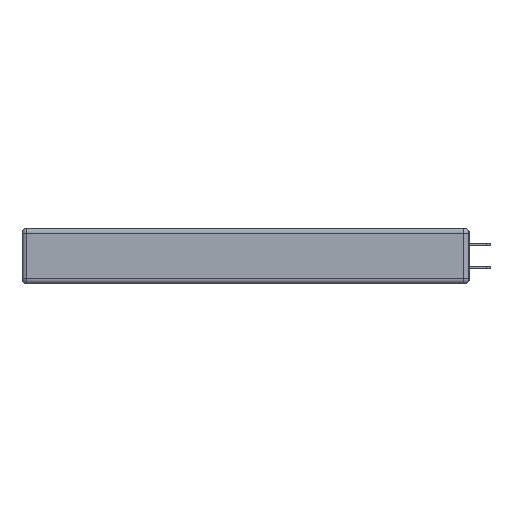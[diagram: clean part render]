
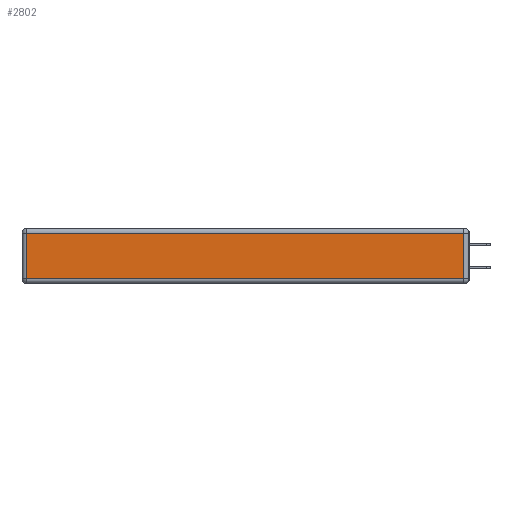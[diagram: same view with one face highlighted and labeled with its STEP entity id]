
A CAD part, left-side view. The second image highlights one B-rep face of the part: STEP entity #2802.
In plain terms, the highlighted planar face has unit normal (-1, 0, 0).
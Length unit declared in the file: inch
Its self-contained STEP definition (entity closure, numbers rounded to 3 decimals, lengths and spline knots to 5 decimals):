
#198 = CARTESIAN_POINT ( 'NONE',  ( 0., 0.03, -0.343 ) ) ;
#644 = VECTOR ( 'NONE', #16991, 39.37008 ) ;
#685 = VERTEX_POINT ( 'NONE', #16792 ) ;
#853 = EDGE_CURVE ( 'NONE', #19598, #13780, #11826, .T. ) ;
#2133 = AXIS2_PLACEMENT_3D ( 'NONE', #5195, #9958, #15181 ) ;
#2802 = ADVANCED_FACE ( 'NONE', ( #8059 ), #3278, .T. ) ;
#2991 = VERTEX_POINT ( 'NONE', #11615 ) ;
#3278 = PLANE ( 'NONE',  #2133 ) ;
#3308 = ORIENTED_EDGE ( 'NONE', *, *, #9346, .T. ) ;
#4881 = EDGE_CURVE ( 'NONE', #2991, #19598, #14632, .T. ) ;
#5195 = CARTESIAN_POINT ( 'NONE',  ( 0., 0., -0.343 ) ) ;
#5577 = LINE ( 'NONE', #198, #13434 ) ;
#5727 = ORIENTED_EDGE ( 'NONE', *, *, #4881, .T. ) ;
#6136 = VECTOR ( 'NONE', #11802, 39.37008 ) ;
#6183 = CARTESIAN_POINT ( 'NONE',  ( 0., 2.72, -0.343 ) ) ;
#6279 = DIRECTION ( 'NONE',  ( 0., 0., 1. ) ) ;
#7828 = LINE ( 'NONE', #13445, #6136 ) ;
#8059 = FACE_OUTER_BOUND ( 'NONE', #19963, .T. ) ;
#9022 = CARTESIAN_POINT ( 'NONE',  ( 0., 2.75, -0.03 ) ) ;
#9346 = EDGE_CURVE ( 'NONE', #685, #2991, #5577, .T. ) ;
#9958 = DIRECTION ( 'NONE',  ( -1., 0., 0. ) ) ;
#10812 = VECTOR ( 'NONE', #17416, 39.37008 ) ;
#11615 = CARTESIAN_POINT ( 'NONE',  ( 0., 0.03, -0.03 ) ) ;
#11802 = DIRECTION ( 'NONE',  ( 0., -1., 0. ) ) ;
#11826 = LINE ( 'NONE', #6183, #10812 ) ;
#13356 = EDGE_CURVE ( 'NONE', #13780, #685, #7828, .T. ) ;
#13434 = VECTOR ( 'NONE', #6279, 39.37008 ) ;
#13445 = CARTESIAN_POINT ( 'NONE',  ( 0., 0., -0.313 ) ) ;
#13780 = VERTEX_POINT ( 'NONE', #19910 ) ;
#14070 = ORIENTED_EDGE ( 'NONE', *, *, #13356, .T. ) ;
#14632 = LINE ( 'NONE', #9022, #644 ) ;
#15013 = CARTESIAN_POINT ( 'NONE',  ( 0., 2.72, -0.03 ) ) ;
#15181 = DIRECTION ( 'NONE',  ( 0., 0., 1. ) ) ;
#16792 = CARTESIAN_POINT ( 'NONE',  ( 0., 0.03, -0.313 ) ) ;
#16991 = DIRECTION ( 'NONE',  ( 0., 1., 0. ) ) ;
#17416 = DIRECTION ( 'NONE',  ( 0., 0., -1. ) ) ;
#19598 = VERTEX_POINT ( 'NONE', #15013 ) ;
#19910 = CARTESIAN_POINT ( 'NONE',  ( 0., 2.72, -0.313 ) ) ;
#19949 = ORIENTED_EDGE ( 'NONE', *, *, #853, .T. ) ;
#19963 = EDGE_LOOP ( 'NONE', ( #14070, #3308, #5727, #19949 ) ) ;
